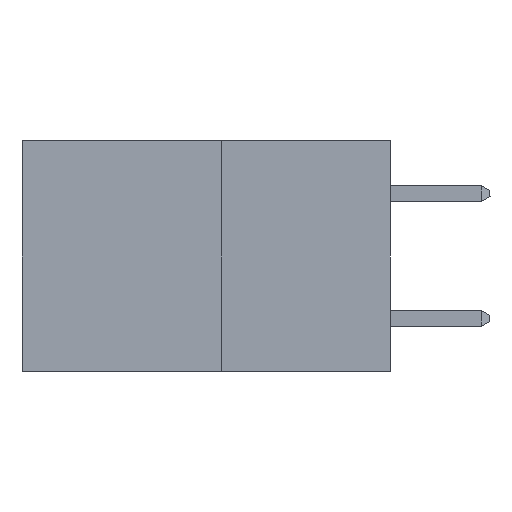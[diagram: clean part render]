
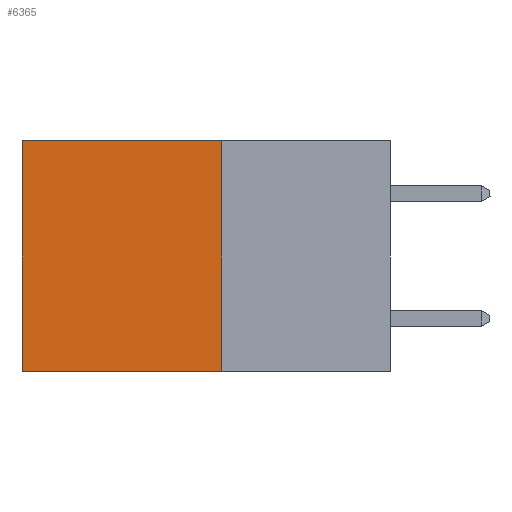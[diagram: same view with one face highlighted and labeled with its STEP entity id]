
A CAD part, left-side view. The second image highlights one B-rep face of the part: STEP entity #6365.
In plain terms, the highlighted planar face has unit normal (-1, 0, 0).
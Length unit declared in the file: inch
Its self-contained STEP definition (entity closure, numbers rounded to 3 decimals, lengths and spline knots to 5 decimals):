
#141 = EDGE_LOOP ( 'NONE', ( #24952, #6449, #12687, #18893 ) ) ;
#1100 = DIRECTION ( 'NONE',  ( 0., 0., -1. ) ) ;
#1296 = DIRECTION ( 'NONE',  ( 1., 0., 0. ) ) ;
#1405 = CARTESIAN_POINT ( 'NONE',  ( 0.277, 0.59, 0. ) ) ;
#2729 = CARTESIAN_POINT ( 'NONE',  ( 0.277, 0.27, -0.37 ) ) ;
#2818 = VECTOR ( 'NONE', #12719, 39.37008 ) ;
#3709 = AXIS2_PLACEMENT_3D ( 'NONE', #24491, #1296, #1100 ) ;
#3715 = EDGE_CURVE ( 'NONE', #18397, #24373, #4370, .T. ) ;
#4370 = LINE ( 'NONE', #31779, #10648 ) ;
#5555 = DIRECTION ( 'NONE',  ( 0., 1., 0. ) ) ;
#6365 = ADVANCED_FACE ( 'NONE', ( #15525 ), #32250, .F. ) ;
#6449 = ORIENTED_EDGE ( 'NONE', *, *, #14950, .F. ) ;
#9213 = CARTESIAN_POINT ( 'NONE',  ( 0.277, 0.27, -0.37 ) ) ;
#10648 = VECTOR ( 'NONE', #31692, 39.37008 ) ;
#12687 = ORIENTED_EDGE ( 'NONE', *, *, #27366, .F. ) ;
#12719 = DIRECTION ( 'NONE',  ( 0., 0., -1. ) ) ;
#14950 = EDGE_CURVE ( 'NONE', #24742, #25007, #22239, .T. ) ;
#15048 = VECTOR ( 'NONE', #22686, 39.37008 ) ;
#15525 = FACE_OUTER_BOUND ( 'NONE', #141, .T. ) ;
#17864 = CARTESIAN_POINT ( 'NONE',  ( 0.277, 0.27, 0. ) ) ;
#18397 = VERTEX_POINT ( 'NONE', #17864 ) ;
#18893 = ORIENTED_EDGE ( 'NONE', *, *, #3715, .T. ) ;
#22188 = LINE ( 'NONE', #9213, #15048 ) ;
#22239 = LINE ( 'NONE', #26787, #28333 ) ;
#22475 = CARTESIAN_POINT ( 'NONE',  ( 0.277, 0.59, -0.37 ) ) ;
#22603 = EDGE_CURVE ( 'NONE', #24373, #25007, #24115, .T. ) ;
#22686 = DIRECTION ( 'NONE',  ( 0., 0., -1. ) ) ;
#24115 = LINE ( 'NONE', #33811, #2818 ) ;
#24373 = VERTEX_POINT ( 'NONE', #1405 ) ;
#24491 = CARTESIAN_POINT ( 'NONE',  ( 0.277, 0.27, -0.37 ) ) ;
#24742 = VERTEX_POINT ( 'NONE', #2729 ) ;
#24952 = ORIENTED_EDGE ( 'NONE', *, *, #22603, .T. ) ;
#25007 = VERTEX_POINT ( 'NONE', #22475 ) ;
#26787 = CARTESIAN_POINT ( 'NONE',  ( 0.277, 0.27, -0.37 ) ) ;
#27366 = EDGE_CURVE ( 'NONE', #18397, #24742, #22188, .T. ) ;
#28333 = VECTOR ( 'NONE', #5555, 39.37008 ) ;
#31692 = DIRECTION ( 'NONE',  ( 0., 1., 0. ) ) ;
#31779 = CARTESIAN_POINT ( 'NONE',  ( 0.277, 0.27, 0. ) ) ;
#32250 = PLANE ( 'NONE',  #3709 ) ;
#33811 = CARTESIAN_POINT ( 'NONE',  ( 0.277, 0.59, -0.37 ) ) ;
